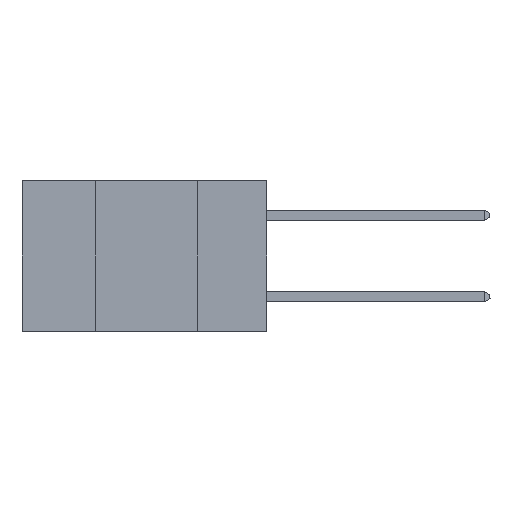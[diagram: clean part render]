
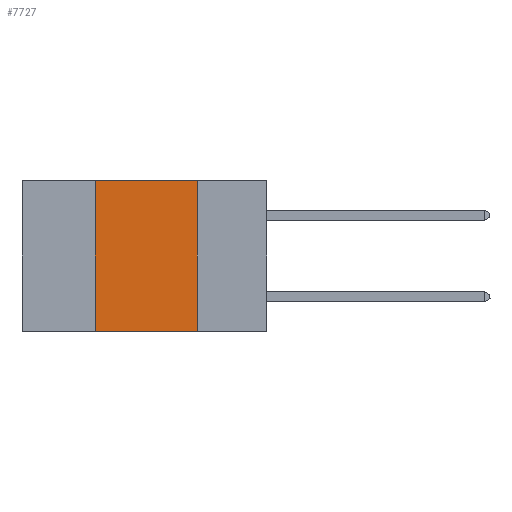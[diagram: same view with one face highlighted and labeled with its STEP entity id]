
A CAD part, left-side view. The second image highlights one B-rep face of the part: STEP entity #7727.
In plain terms, the highlighted planar face has unit normal (-1, 0, 0).
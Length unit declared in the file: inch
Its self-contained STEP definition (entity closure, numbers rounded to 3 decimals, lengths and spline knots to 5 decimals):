
#397 = LINE ( 'NONE', #15747, #3227 ) ;
#950 = EDGE_CURVE ( 'NONE', #12745, #23074, #397, .T. ) ;
#1723 = ORIENTED_EDGE ( 'NONE', *, *, #8182, .F. ) ;
#3227 = VECTOR ( 'NONE', #17508, 39.37008 ) ;
#3962 = CARTESIAN_POINT ( 'NONE',  ( 0., 0.42, 0. ) ) ;
#4570 = VECTOR ( 'NONE', #8093, 39.37008 ) ;
#4694 = DIRECTION ( 'NONE',  ( 0., 0., -1. ) ) ;
#5414 = ORIENTED_EDGE ( 'NONE', *, *, #16923, .F. ) ;
#5444 = VECTOR ( 'NONE', #4694, 39.37008 ) ;
#7008 = FACE_OUTER_BOUND ( 'NONE', #10171, .T. ) ;
#7727 = ADVANCED_FACE ( 'NONE', ( #7008 ), #17437, .F. ) ;
#8018 = DIRECTION ( 'NONE',  ( 0., -1., 0. ) ) ;
#8093 = DIRECTION ( 'NONE',  ( 0., -1., 0. ) ) ;
#8182 = EDGE_CURVE ( 'NONE', #22779, #8403, #12001, .T. ) ;
#8403 = VERTEX_POINT ( 'NONE', #17667 ) ;
#8599 = AXIS2_PLACEMENT_3D ( 'NONE', #21736, #9617, #9438 ) ;
#9438 = DIRECTION ( 'NONE',  ( 0., 0., -1. ) ) ;
#9617 = DIRECTION ( 'NONE',  ( 1., 0., 0. ) ) ;
#9893 = LINE ( 'NONE', #18220, #4570 ) ;
#10171 = EDGE_LOOP ( 'NONE', ( #1723, #5414, #15140, #22228 ) ) ;
#10295 = LINE ( 'NONE', #22166, #11237 ) ;
#11237 = VECTOR ( 'NONE', #8018, 39.37008 ) ;
#12001 = LINE ( 'NONE', #22863, #5444 ) ;
#12745 = VERTEX_POINT ( 'NONE', #22259 ) ;
#14204 = EDGE_CURVE ( 'NONE', #12745, #8403, #10295, .T. ) ;
#15140 = ORIENTED_EDGE ( 'NONE', *, *, #950, .F. ) ;
#15747 = CARTESIAN_POINT ( 'NONE',  ( 0., 0.42, 0. ) ) ;
#16923 = EDGE_CURVE ( 'NONE', #23074, #22779, #9893, .T. ) ;
#17210 = CARTESIAN_POINT ( 'NONE',  ( 0., 0.17, 0. ) ) ;
#17437 = PLANE ( 'NONE',  #8599 ) ;
#17508 = DIRECTION ( 'NONE',  ( 0., 0., 1. ) ) ;
#17667 = CARTESIAN_POINT ( 'NONE',  ( 0., 0.17, -0.37 ) ) ;
#18220 = CARTESIAN_POINT ( 'NONE',  ( 0., 0.6, 0. ) ) ;
#21736 = CARTESIAN_POINT ( 'NONE',  ( 0., 0.6, 0. ) ) ;
#22166 = CARTESIAN_POINT ( 'NONE',  ( 0., 0.6, -0.37 ) ) ;
#22228 = ORIENTED_EDGE ( 'NONE', *, *, #14204, .T. ) ;
#22259 = CARTESIAN_POINT ( 'NONE',  ( 0., 0.42, -0.37 ) ) ;
#22779 = VERTEX_POINT ( 'NONE', #17210 ) ;
#22863 = CARTESIAN_POINT ( 'NONE',  ( 0., 0.17, 0. ) ) ;
#23074 = VERTEX_POINT ( 'NONE', #3962 ) ;
